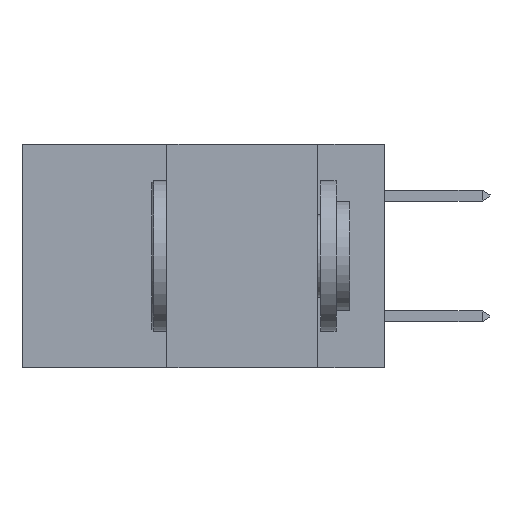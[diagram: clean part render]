
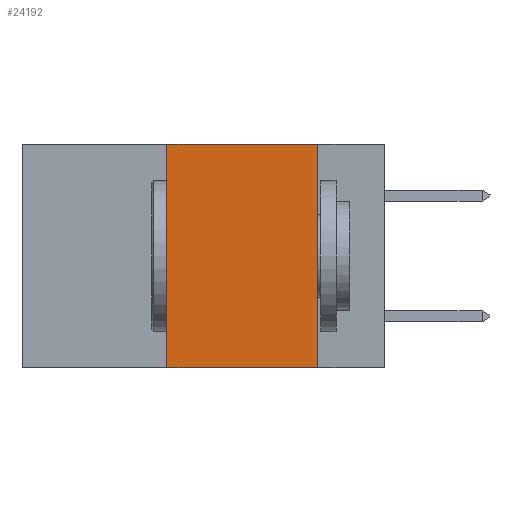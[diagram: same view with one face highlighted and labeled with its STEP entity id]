
A CAD part, left-side view. The second image highlights one B-rep face of the part: STEP entity #24192.
In plain terms, the highlighted planar face has unit normal (-1, 0, 0).
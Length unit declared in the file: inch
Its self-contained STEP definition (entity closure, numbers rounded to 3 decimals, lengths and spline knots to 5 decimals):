
#570 = DIRECTION ( 'NONE',  ( 0., 0., -1. ) ) ;
#2428 = ORIENTED_EDGE ( 'NONE', *, *, #26499, .F. ) ;
#3103 = ORIENTED_EDGE ( 'NONE', *, *, #24868, .F. ) ;
#3605 = LINE ( 'NONE', #36151, #29489 ) ;
#3794 = AXIS2_PLACEMENT_3D ( 'NONE', #30847, #20860, #570 ) ;
#5390 = VERTEX_POINT ( 'NONE', #19271 ) ;
#6748 = CARTESIAN_POINT ( 'NONE',  ( 0., 0.6, -0.37 ) ) ;
#9440 = CARTESIAN_POINT ( 'NONE',  ( 0., 0.36, 0. ) ) ;
#10362 = VERTEX_POINT ( 'NONE', #26485 ) ;
#13985 = DIRECTION ( 'NONE',  ( 0., 0., -1. ) ) ;
#14198 = ORIENTED_EDGE ( 'NONE', *, *, #38897, .F. ) ;
#15847 = VERTEX_POINT ( 'NONE', #16051 ) ;
#16014 = DIRECTION ( 'NONE',  ( 0., -1., 0. ) ) ;
#16051 = CARTESIAN_POINT ( 'NONE',  ( 0., 0.36, -0.37 ) ) ;
#16605 = EDGE_CURVE ( 'NONE', #15847, #5390, #33321, .T. ) ;
#17010 = DIRECTION ( 'NONE',  ( 0., -1., 0. ) ) ;
#17212 = LINE ( 'NONE', #17428, #33999 ) ;
#17305 = ORIENTED_EDGE ( 'NONE', *, *, #16605, .T. ) ;
#17428 = CARTESIAN_POINT ( 'NONE',  ( 0., 0.11, 0. ) ) ;
#17479 = PLANE ( 'NONE',  #3794 ) ;
#19271 = CARTESIAN_POINT ( 'NONE',  ( 0., 0.11, -0.37 ) ) ;
#20860 = DIRECTION ( 'NONE',  ( 1., 0., 0. ) ) ;
#21003 = LINE ( 'NONE', #9440, #27826 ) ;
#24192 = ADVANCED_FACE ( 'NONE', ( #35645 ), #17479, .F. ) ;
#24868 = EDGE_CURVE ( 'NONE', #10362, #5390, #17212, .T. ) ;
#26485 = CARTESIAN_POINT ( 'NONE',  ( 0., 0.11, 0. ) ) ;
#26499 = EDGE_CURVE ( 'NONE', #15847, #42186, #21003, .T. ) ;
#27826 = VECTOR ( 'NONE', #39655, 39.37008 ) ;
#29489 = VECTOR ( 'NONE', #16014, 39.37008 ) ;
#30847 = CARTESIAN_POINT ( 'NONE',  ( 0., 0.6, 0. ) ) ;
#31214 = VECTOR ( 'NONE', #17010, 39.37008 ) ;
#32420 = EDGE_LOOP ( 'NONE', ( #3103, #14198, #2428, #17305 ) ) ;
#33321 = LINE ( 'NONE', #6748, #31214 ) ;
#33999 = VECTOR ( 'NONE', #13985, 39.37008 ) ;
#35645 = FACE_OUTER_BOUND ( 'NONE', #32420, .T. ) ;
#36151 = CARTESIAN_POINT ( 'NONE',  ( 0., 0.6, 0. ) ) ;
#38897 = EDGE_CURVE ( 'NONE', #42186, #10362, #3605, .T. ) ;
#39655 = DIRECTION ( 'NONE',  ( 0., 0., 1. ) ) ;
#41027 = CARTESIAN_POINT ( 'NONE',  ( 0., 0.36, 0. ) ) ;
#42186 = VERTEX_POINT ( 'NONE', #41027 ) ;
